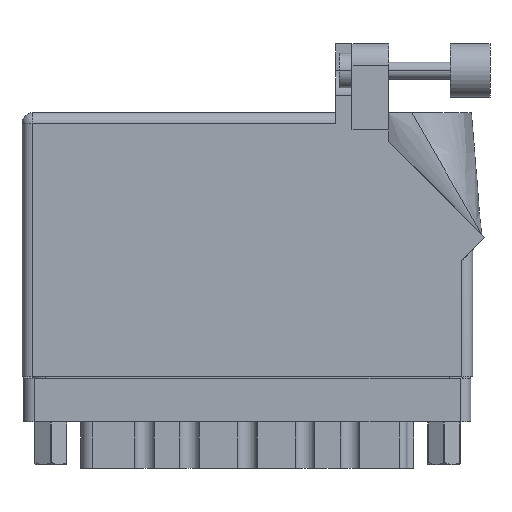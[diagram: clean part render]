
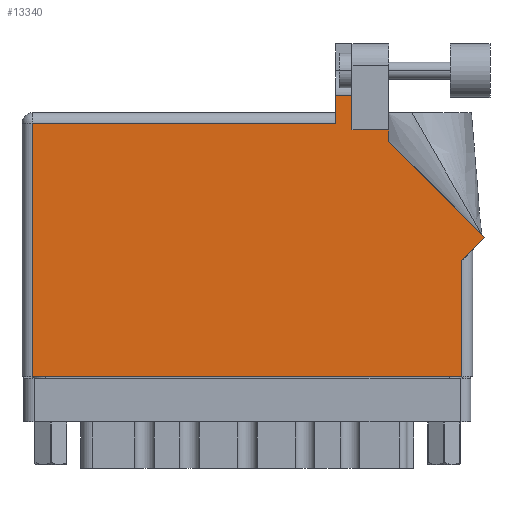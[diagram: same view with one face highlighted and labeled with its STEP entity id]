
A CAD part, front view. The second image highlights one B-rep face of the part: STEP entity #13340.
In plain terms, the highlighted face is planar.
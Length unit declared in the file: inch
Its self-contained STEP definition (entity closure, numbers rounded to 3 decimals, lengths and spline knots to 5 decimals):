
#524 = CARTESIAN_POINT ( 'NONE',  ( 0., 1.53, 0. ) ) ;
#543 = CARTESIAN_POINT ( 'NONE',  ( 2.126, 1.43, 0. ) ) ;
#1124 = DIRECTION ( 'NONE',  ( -1., 0., 0. ) ) ;
#1498 = CARTESIAN_POINT ( 'NONE',  ( 2.55, 0.675, 0. ) ) ;
#1663 = ORIENTED_EDGE ( 'NONE', *, *, #14737, .T. ) ;
#2209 = EDGE_CURVE ( 'NONE', #31207, #37691, #21618, .T. ) ;
#2380 = CARTESIAN_POINT ( 'NONE',  ( 1.913, 1.43, 0. ) ) ;
#2786 = CARTESIAN_POINT ( 'NONE',  ( 2.126, 1.36442, 0. ) ) ;
#3175 = CARTESIAN_POINT ( 'NONE',  ( 1.819, 1.468, 0. ) ) ;
#4292 = EDGE_CURVE ( 'NONE', #33538, #4587, #4438, .T. ) ;
#4361 = VERTEX_POINT ( 'NONE', #52367 ) ;
#4399 = VERTEX_POINT ( 'NONE', #31995 ) ;
#4438 = LINE ( 'NONE', #16522, #57008 ) ;
#4587 = VERTEX_POINT ( 'NONE', #28495 ) ;
#4802 = DIRECTION ( 'NONE',  ( 1., 0., 0. ) ) ;
#5281 = CARTESIAN_POINT ( 'NONE',  ( 2.612, 0.737, 0. ) ) ;
#6418 = CARTESIAN_POINT ( 'NONE',  ( 0.062, 0., 0. ) ) ;
#8269 = LINE ( 'NONE', #18797, #48929 ) ;
#8516 = EDGE_CURVE ( 'NONE', #54157, #40328, #8269, .T. ) ;
#9744 = PLANE ( 'NONE',  #18945 ) ;
#11839 = LINE ( 'NONE', #5281, #34402 ) ;
#11995 = CARTESIAN_POINT ( 'NONE',  ( 1.819, 1.53, 0. ) ) ;
#13302 = EDGE_LOOP ( 'NONE', ( #28070, #40367, #27518, #28256, #51311, #47740, #47037, #1663, #44046, #30149, #38581 ) ) ;
#13340 = ADVANCED_FACE ( 'NONE', ( #33768 ), #9744, .F. ) ;
#14737 = EDGE_CURVE ( 'NONE', #37691, #4361, #11839, .T. ) ;
#14765 = DIRECTION ( 'NONE',  ( -1., 0., 0. ) ) ;
#15026 = CARTESIAN_POINT ( 'NONE',  ( 1.819, 1.6315, 0. ) ) ;
#15176 = LINE ( 'NONE', #41679, #52370 ) ;
#15478 = CARTESIAN_POINT ( 'NONE',  ( 2.55, 0.737, 0. ) ) ;
#15950 = VERTEX_POINT ( 'NONE', #15026 ) ;
#16522 = CARTESIAN_POINT ( 'NONE',  ( 1.913, 1.43, 0. ) ) ;
#16862 = EDGE_CURVE ( 'NONE', #4399, #31207, #55818, .T. ) ;
#16935 = VERTEX_POINT ( 'NONE', #17962 ) ;
#17962 = CARTESIAN_POINT ( 'NONE',  ( 0.062, 1.468, 0. ) ) ;
#18797 = CARTESIAN_POINT ( 'NONE',  ( 2.126, 1.36442, 0. ) ) ;
#18945 = AXIS2_PLACEMENT_3D ( 'NONE', #524, #50131, #27265 ) ;
#18967 = VERTEX_POINT ( 'NONE', #3175 ) ;
#18975 = EDGE_CURVE ( 'NONE', #15950, #18967, #37765, .T. ) ;
#20041 = EDGE_CURVE ( 'NONE', #16935, #4399, #31382, .T. ) ;
#21618 = LINE ( 'NONE', #15478, #53158 ) ;
#23329 = EDGE_CURVE ( 'NONE', #4361, #54157, #35844, .T. ) ;
#23533 = DIRECTION ( 'NONE',  ( 0., 1., 0. ) ) ;
#24961 = LINE ( 'NONE', #36833, #45296 ) ;
#25742 = VECTOR ( 'NONE', #27655, 39.37008 ) ;
#27054 = VECTOR ( 'NONE', #4802, 39.37008 ) ;
#27265 = DIRECTION ( 'NONE',  ( -1., 0., 0. ) ) ;
#27518 = ORIENTED_EDGE ( 'NONE', *, *, #18975, .T. ) ;
#27655 = DIRECTION ( 'NONE',  ( -1., 0., 0. ) ) ;
#28070 = ORIENTED_EDGE ( 'NONE', *, *, #4292, .T. ) ;
#28256 = ORIENTED_EDGE ( 'NONE', *, *, #31404, .T. ) ;
#28495 = CARTESIAN_POINT ( 'NONE',  ( 1.913, 1.6315, 0. ) ) ;
#30149 = ORIENTED_EDGE ( 'NONE', *, *, #8516, .T. ) ;
#31207 = VERTEX_POINT ( 'NONE', #33415 ) ;
#31382 = LINE ( 'NONE', #6418, #53779 ) ;
#31404 = EDGE_CURVE ( 'NONE', #18967, #16935, #24961, .T. ) ;
#31526 = DIRECTION ( 'NONE',  ( -0.707, 0.707, 0. ) ) ;
#31995 = CARTESIAN_POINT ( 'NONE',  ( 0.062, 0., 0. ) ) ;
#33415 = CARTESIAN_POINT ( 'NONE',  ( 2.55, 0., 0. ) ) ;
#33538 = VERTEX_POINT ( 'NONE', #2380 ) ;
#33768 = FACE_OUTER_BOUND ( 'NONE', #13302, .T. ) ;
#34402 = VECTOR ( 'NONE', #41372, 39.37008 ) ;
#34540 = EDGE_CURVE ( 'NONE', #4587, #15950, #42588, .T. ) ;
#35844 = LINE ( 'NONE', #53837, #51320 ) ;
#36833 = CARTESIAN_POINT ( 'NONE',  ( 0., 1.468, 0. ) ) ;
#37678 = DIRECTION ( 'NONE',  ( 0., 1., 0. ) ) ;
#37691 = VERTEX_POINT ( 'NONE', #1498 ) ;
#37765 = LINE ( 'NONE', #11995, #46137 ) ;
#38581 = ORIENTED_EDGE ( 'NONE', *, *, #55852, .T. ) ;
#40328 = VERTEX_POINT ( 'NONE', #543 ) ;
#40367 = ORIENTED_EDGE ( 'NONE', *, *, #34540, .T. ) ;
#41372 = DIRECTION ( 'NONE',  ( 0.707, 0.707, 0. ) ) ;
#41679 = CARTESIAN_POINT ( 'NONE',  ( 2.126, 1.43, 0. ) ) ;
#42588 = LINE ( 'NONE', #45635, #25742 ) ;
#42719 = DIRECTION ( 'NONE',  ( 0., -1., 0. ) ) ;
#44046 = ORIENTED_EDGE ( 'NONE', *, *, #23329, .T. ) ;
#45296 = VECTOR ( 'NONE', #1124, 39.37008 ) ;
#45635 = CARTESIAN_POINT ( 'NONE',  ( 2.24377, 1.6315, 0. ) ) ;
#46137 = VECTOR ( 'NONE', #47904, 39.37008 ) ;
#47037 = ORIENTED_EDGE ( 'NONE', *, *, #2209, .T. ) ;
#47740 = ORIENTED_EDGE ( 'NONE', *, *, #16862, .T. ) ;
#47904 = DIRECTION ( 'NONE',  ( 0., -1., 0. ) ) ;
#48929 = VECTOR ( 'NONE', #23533, 39.37008 ) ;
#50131 = DIRECTION ( 'NONE',  ( 0., 0., -1. ) ) ;
#51311 = ORIENTED_EDGE ( 'NONE', *, *, #20041, .T. ) ;
#51320 = VECTOR ( 'NONE', #31526, 39.37008 ) ;
#52367 = CARTESIAN_POINT ( 'NONE',  ( 2.68271, 0.80771, 0. ) ) ;
#52370 = VECTOR ( 'NONE', #14765, 39.37008 ) ;
#52568 = DIRECTION ( 'NONE',  ( 0., 1., 0. ) ) ;
#53158 = VECTOR ( 'NONE', #37678, 39.37008 ) ;
#53653 = CARTESIAN_POINT ( 'NONE',  ( 0., 0., 0. ) ) ;
#53779 = VECTOR ( 'NONE', #42719, 39.37008 ) ;
#53837 = CARTESIAN_POINT ( 'NONE',  ( 2.68271, 0.80771, 0. ) ) ;
#54157 = VERTEX_POINT ( 'NONE', #2786 ) ;
#55818 = LINE ( 'NONE', #53653, #27054 ) ;
#55852 = EDGE_CURVE ( 'NONE', #40328, #33538, #15176, .T. ) ;
#57008 = VECTOR ( 'NONE', #52568, 39.37008 ) ;
